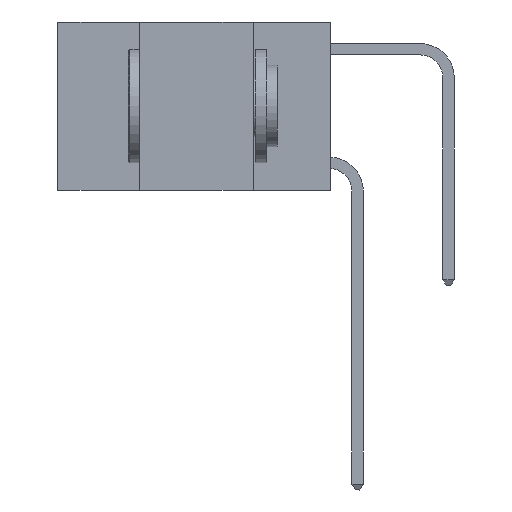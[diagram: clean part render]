
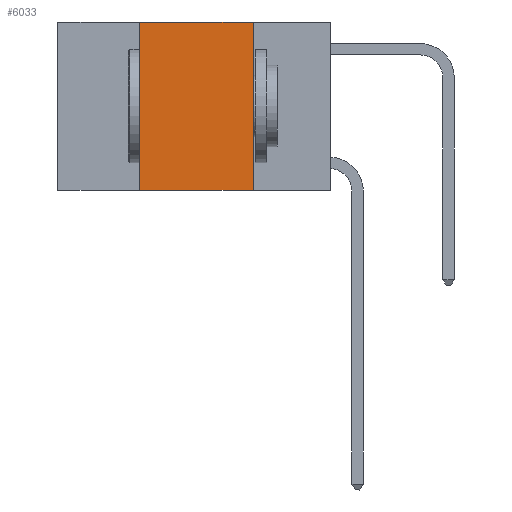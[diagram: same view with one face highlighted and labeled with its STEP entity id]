
A CAD part, left-side view. The second image highlights one B-rep face of the part: STEP entity #6033.
In plain terms, the highlighted planar face has unit normal (-1, 0, 0).
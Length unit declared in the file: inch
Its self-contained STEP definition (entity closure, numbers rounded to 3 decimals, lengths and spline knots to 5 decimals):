
#194 = VERTEX_POINT ( 'NONE', #11215 ) ;
#524 = DIRECTION ( 'NONE',  ( 1., 0., 0. ) ) ;
#682 = VERTEX_POINT ( 'NONE', #13812 ) ;
#983 = VECTOR ( 'NONE', #8450, 39.37008 ) ;
#1090 = LINE ( 'NONE', #2982, #9791 ) ;
#1149 = VERTEX_POINT ( 'NONE', #9754 ) ;
#1328 = EDGE_CURVE ( 'NONE', #8292, #194, #2770, .T. ) ;
#1561 = LINE ( 'NONE', #3733, #2223 ) ;
#1876 = EDGE_CURVE ( 'NONE', #194, #682, #1561, .T. ) ;
#2115 = LINE ( 'NONE', #4127, #983 ) ;
#2223 = VECTOR ( 'NONE', #5818, 39.37008 ) ;
#2696 = DIRECTION ( 'NONE',  ( 0., -1., 0. ) ) ;
#2770 = LINE ( 'NONE', #11080, #6287 ) ;
#2830 = DIRECTION ( 'NONE',  ( 0., 0., -1. ) ) ;
#2982 = CARTESIAN_POINT ( 'NONE',  ( 0., 0.42, 0. ) ) ;
#3247 = EDGE_CURVE ( 'NONE', #1149, #682, #2115, .T. ) ;
#3733 = CARTESIAN_POINT ( 'NONE',  ( 0., 0.17, 0. ) ) ;
#4127 = CARTESIAN_POINT ( 'NONE',  ( 0., 0.6, -0.37 ) ) ;
#4900 = AXIS2_PLACEMENT_3D ( 'NONE', #8171, #524, #2830 ) ;
#5818 = DIRECTION ( 'NONE',  ( 0., 0., -1. ) ) ;
#6033 = ADVANCED_FACE ( 'NONE', ( #10275 ), #13268, .F. ) ;
#6220 = ORIENTED_EDGE ( 'NONE', *, *, #1876, .F. ) ;
#6287 = VECTOR ( 'NONE', #2696, 39.37008 ) ;
#6551 = ORIENTED_EDGE ( 'NONE', *, *, #3247, .T. ) ;
#6913 = EDGE_LOOP ( 'NONE', ( #6220, #11322, #13283, #6551 ) ) ;
#8058 = CARTESIAN_POINT ( 'NONE',  ( 0., 0.42, 0. ) ) ;
#8171 = CARTESIAN_POINT ( 'NONE',  ( 0., 0.6, 0. ) ) ;
#8292 = VERTEX_POINT ( 'NONE', #8058 ) ;
#8450 = DIRECTION ( 'NONE',  ( 0., -1., 0. ) ) ;
#8914 = EDGE_CURVE ( 'NONE', #1149, #8292, #1090, .T. ) ;
#9754 = CARTESIAN_POINT ( 'NONE',  ( 0., 0.42, -0.37 ) ) ;
#9791 = VECTOR ( 'NONE', #10660, 39.37008 ) ;
#10275 = FACE_OUTER_BOUND ( 'NONE', #6913, .T. ) ;
#10660 = DIRECTION ( 'NONE',  ( 0., 0., 1. ) ) ;
#11080 = CARTESIAN_POINT ( 'NONE',  ( 0., 0.6, 0. ) ) ;
#11215 = CARTESIAN_POINT ( 'NONE',  ( 0., 0.17, 0. ) ) ;
#11322 = ORIENTED_EDGE ( 'NONE', *, *, #1328, .F. ) ;
#13268 = PLANE ( 'NONE',  #4900 ) ;
#13283 = ORIENTED_EDGE ( 'NONE', *, *, #8914, .F. ) ;
#13812 = CARTESIAN_POINT ( 'NONE',  ( 0., 0.17, -0.37 ) ) ;
